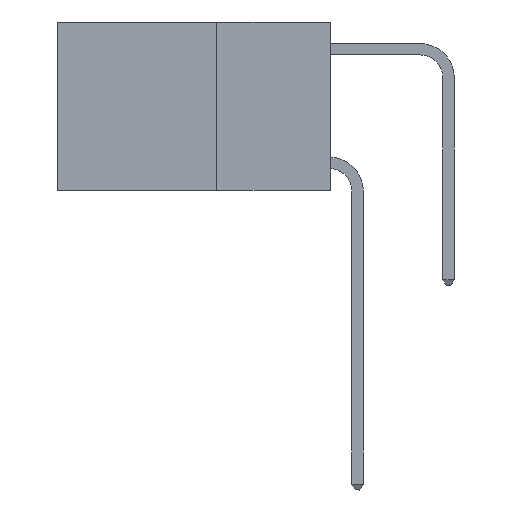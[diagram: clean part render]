
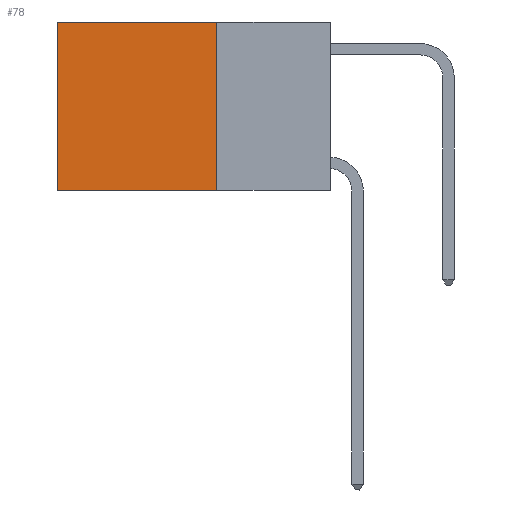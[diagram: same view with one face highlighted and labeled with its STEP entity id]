
A CAD part, left-side view. The second image highlights one B-rep face of the part: STEP entity #78.
In plain terms, the highlighted planar face has unit normal (-1, 0, 0).
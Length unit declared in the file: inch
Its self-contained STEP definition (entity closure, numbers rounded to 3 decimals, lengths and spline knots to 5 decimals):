
#78 = ADVANCED_FACE ( 'NONE', ( #10567 ), #6585, .F. ) ;
#584 = EDGE_CURVE ( 'NONE', #25145, #4455, #24804, .T. ) ;
#811 = AXIS2_PLACEMENT_3D ( 'NONE', #2552, #18359, #6426 ) ;
#1916 = LINE ( 'NONE', #21990, #22331 ) ;
#2325 = EDGE_CURVE ( 'NONE', #21140, #25000, #24424, .T. ) ;
#2552 = CARTESIAN_POINT ( 'NONE',  ( 0.2625, 0.25, 0. ) ) ;
#2970 = LINE ( 'NONE', #11566, #16593 ) ;
#4364 = CARTESIAN_POINT ( 'NONE',  ( 0.2625, 0.25, -0.37 ) ) ;
#4455 = VERTEX_POINT ( 'NONE', #18990 ) ;
#5199 = EDGE_LOOP ( 'NONE', ( #11226, #10900, #10610, #14480 ) ) ;
#5806 = DIRECTION ( 'NONE',  ( 0., 1., 0. ) ) ;
#6426 = DIRECTION ( 'NONE',  ( 0., 0., -1. ) ) ;
#6585 = PLANE ( 'NONE',  #811 ) ;
#8193 = EDGE_CURVE ( 'NONE', #21140, #25145, #1916, .T. ) ;
#9834 = CARTESIAN_POINT ( 'NONE',  ( 0.2625, 0.6, 0. ) ) ;
#9876 = VECTOR ( 'NONE', #5806, 39.37008 ) ;
#10567 = FACE_OUTER_BOUND ( 'NONE', #5199, .T. ) ;
#10610 = ORIENTED_EDGE ( 'NONE', *, *, #8193, .F. ) ;
#10900 = ORIENTED_EDGE ( 'NONE', *, *, #584, .F. ) ;
#11001 = CARTESIAN_POINT ( 'NONE',  ( 0.2625, 0.25, 0. ) ) ;
#11226 = ORIENTED_EDGE ( 'NONE', *, *, #20048, .T. ) ;
#11467 = VECTOR ( 'NONE', #22240, 39.37008 ) ;
#11566 = CARTESIAN_POINT ( 'NONE',  ( 0.2625, 0.6, 0. ) ) ;
#14480 = ORIENTED_EDGE ( 'NONE', *, *, #2325, .T. ) ;
#15607 = CARTESIAN_POINT ( 'NONE',  ( 0.2625, 0.25, 0. ) ) ;
#16175 = CARTESIAN_POINT ( 'NONE',  ( 0.2625, 0.25, -0.37 ) ) ;
#16593 = VECTOR ( 'NONE', #17847, 39.37008 ) ;
#17847 = DIRECTION ( 'NONE',  ( 0., 0., -1. ) ) ;
#18359 = DIRECTION ( 'NONE',  ( 1., 0., 0. ) ) ;
#18990 = CARTESIAN_POINT ( 'NONE',  ( 0.2625, 0.6, -0.37 ) ) ;
#20048 = EDGE_CURVE ( 'NONE', #25000, #4455, #2970, .T. ) ;
#21140 = VERTEX_POINT ( 'NONE', #11001 ) ;
#21990 = CARTESIAN_POINT ( 'NONE',  ( 0.2625, 0.25, 0. ) ) ;
#22240 = DIRECTION ( 'NONE',  ( 0., 1., 0. ) ) ;
#22331 = VECTOR ( 'NONE', #23646, 39.37008 ) ;
#23646 = DIRECTION ( 'NONE',  ( 0., 0., -1. ) ) ;
#24424 = LINE ( 'NONE', #15607, #9876 ) ;
#24804 = LINE ( 'NONE', #16175, #11467 ) ;
#25000 = VERTEX_POINT ( 'NONE', #9834 ) ;
#25145 = VERTEX_POINT ( 'NONE', #4364 ) ;
